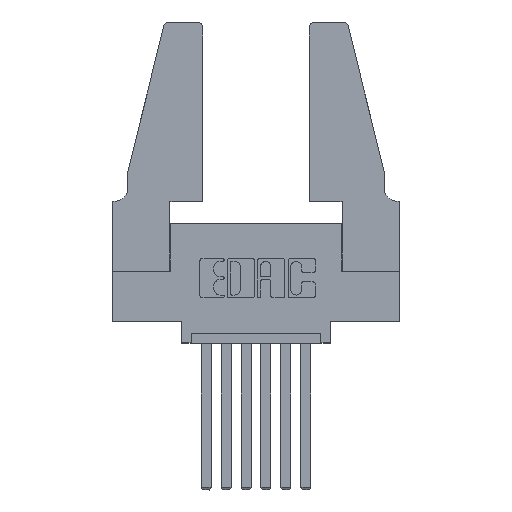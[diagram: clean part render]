
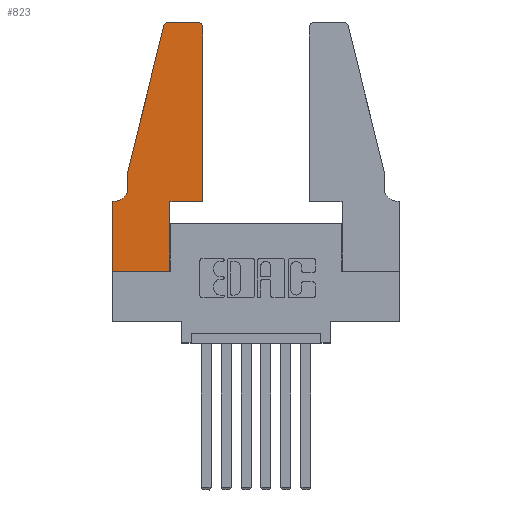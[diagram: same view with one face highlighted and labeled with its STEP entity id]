
A CAD part, top view. The second image highlights one B-rep face of the part: STEP entity #823.
In plain terms, the highlighted planar face has unit normal (0, 0, 1).
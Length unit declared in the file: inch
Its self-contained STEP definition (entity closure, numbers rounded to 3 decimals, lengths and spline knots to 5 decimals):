
#442 = LINE ( 'NONE', #8422, #3242 ) ;
#522 = EDGE_CURVE ( 'NONE', #2364, #3418, #5829, .T. ) ;
#600 = PLANE ( 'NONE',  #9543 ) ;
#605 = EDGE_CURVE ( 'NONE', #1184, #9651, #3217, .T. ) ;
#698 = CARTESIAN_POINT ( 'NONE',  ( 0.4505, 0.35, 0.37 ) ) ;
#705 = DIRECTION ( 'NONE',  ( 1., 0., 0. ) ) ;
#805 = ORIENTED_EDGE ( 'NONE', *, *, #5614, .T. ) ;
#823 = ADVANCED_FACE ( 'NONE', ( #4710 ), #600, .T. ) ;
#920 = CARTESIAN_POINT ( 'NONE',  ( 0.0055, 0.42, 0.37 ) ) ;
#1025 = DIRECTION ( 'NONE',  ( 0., 0., 1. ) ) ;
#1041 = VECTOR ( 'NONE', #3894, 39.37008 ) ;
#1184 = VERTEX_POINT ( 'NONE', #3946 ) ;
#1202 = ORIENTED_EDGE ( 'NONE', *, *, #522, .T. ) ;
#1236 = EDGE_LOOP ( 'NONE', ( #1202, #2286, #8239, #10506, #7059, #2358, #10195, #8709, #805, #8279, #3231, #5158 ) ) ;
#1479 = LINE ( 'NONE', #3176, #9645 ) ;
#1609 = DIRECTION ( 'NONE',  ( -0.239, -0.971, 0. ) ) ;
#1748 = AXIS2_PLACEMENT_3D ( 'NONE', #2645, #4432, #5366 ) ;
#1759 = CARTESIAN_POINT ( 'NONE',  ( 0.0755, 0.5, 0.37 ) ) ;
#1857 = VERTEX_POINT ( 'NONE', #6319 ) ;
#2286 = ORIENTED_EDGE ( 'NONE', *, *, #5593, .T. ) ;
#2358 = ORIENTED_EDGE ( 'NONE', *, *, #8262, .T. ) ;
#2364 = VERTEX_POINT ( 'NONE', #5955 ) ;
#2372 = DIRECTION ( 'NONE',  ( 0., 0., 1. ) ) ;
#2502 = LINE ( 'NONE', #9892, #9300 ) ;
#2555 = CARTESIAN_POINT ( 'NONE',  ( 0.2865, 0., 0.37 ) ) ;
#2618 = CARTESIAN_POINT ( 'NONE',  ( 0.0055, 0.35, 0.37 ) ) ;
#2628 = LINE ( 'NONE', #5241, #9415 ) ;
#2645 = CARTESIAN_POINT ( 'NONE',  ( 0.4205, 1.22, 0.37 ) ) ;
#2779 = VECTOR ( 'NONE', #4278, 39.37008 ) ;
#2802 = CARTESIAN_POINT ( 'NONE',  ( 0.4505, 0.35, 0.37 ) ) ;
#2878 = EDGE_CURVE ( 'NONE', #7506, #5912, #8418, .T. ) ;
#2885 = CARTESIAN_POINT ( 'NONE',  ( 0.284, 1.25, 0.37 ) ) ;
#2950 = EDGE_CURVE ( 'NONE', #1857, #10022, #6340, .T. ) ;
#3176 = CARTESIAN_POINT ( 'NONE',  ( 0., 0., 0.37 ) ) ;
#3217 = LINE ( 'NONE', #698, #2779 ) ;
#3231 = ORIENTED_EDGE ( 'NONE', *, *, #3280, .T. ) ;
#3242 = VECTOR ( 'NONE', #6685, 39.37008 ) ;
#3280 = EDGE_CURVE ( 'NONE', #9651, #7322, #8269, .T. ) ;
#3418 = VERTEX_POINT ( 'NONE', #2885 ) ;
#3425 = CIRCLE ( 'NONE', #10325, 0.03 ) ;
#3571 = VECTOR ( 'NONE', #8111, 39.37008 ) ;
#3894 = DIRECTION ( 'NONE',  ( 0., 1., 0. ) ) ;
#3896 = CARTESIAN_POINT ( 'NONE',  ( 0.4505, 0.35, 0.37 ) ) ;
#3946 = CARTESIAN_POINT ( 'NONE',  ( 0.2865, 0.35, 0.37 ) ) ;
#3966 = DIRECTION ( 'NONE',  ( 1., 0., 0. ) ) ;
#4278 = DIRECTION ( 'NONE',  ( 1., 0., 0. ) ) ;
#4323 = CARTESIAN_POINT ( 'NONE',  ( 0.4505, 1.22, 0.37 ) ) ;
#4432 = DIRECTION ( 'NONE',  ( 0., 0., 1. ) ) ;
#4511 = CARTESIAN_POINT ( 'NONE',  ( 0., 0.35, 0.37 ) ) ;
#4710 = FACE_OUTER_BOUND ( 'NONE', #1236, .T. ) ;
#4759 = VERTEX_POINT ( 'NONE', #4511 ) ;
#5003 = EDGE_CURVE ( 'NONE', #5912, #1857, #442, .T. ) ;
#5158 = ORIENTED_EDGE ( 'NONE', *, *, #9045, .T. ) ;
#5241 = CARTESIAN_POINT ( 'NONE',  ( 0., 0., 0.37 ) ) ;
#5366 = DIRECTION ( 'NONE',  ( 1., 0., 0. ) ) ;
#5539 = VECTOR ( 'NONE', #6517, 39.37008 ) ;
#5593 = EDGE_CURVE ( 'NONE', #3418, #7506, #3425, .T. ) ;
#5614 = EDGE_CURVE ( 'NONE', #10525, #1184, #9784, .T. ) ;
#5745 = CARTESIAN_POINT ( 'NONE',  ( 0.2865, 0.35, 0.37 ) ) ;
#5829 = LINE ( 'NONE', #8240, #5539 ) ;
#5912 = VERTEX_POINT ( 'NONE', #7587 ) ;
#5955 = CARTESIAN_POINT ( 'NONE',  ( 0.4205, 1.25, 0.37 ) ) ;
#6010 = EDGE_CURVE ( 'NONE', #4759, #7731, #1479, .T. ) ;
#6212 = DIRECTION ( 'NONE',  ( -1., 0., 0. ) ) ;
#6319 = CARTESIAN_POINT ( 'NONE',  ( 0.0755, 0.42, 0.37 ) ) ;
#6340 = CIRCLE ( 'NONE', #10141, 0.07 ) ;
#6517 = DIRECTION ( 'NONE',  ( -1., 0., 0. ) ) ;
#6685 = DIRECTION ( 'NONE',  ( 0., -1., 0. ) ) ;
#7049 = CARTESIAN_POINT ( 'NONE',  ( 0., 0., 0.37 ) ) ;
#7059 = ORIENTED_EDGE ( 'NONE', *, *, #2950, .T. ) ;
#7322 = VERTEX_POINT ( 'NONE', #4323 ) ;
#7506 = VERTEX_POINT ( 'NONE', #11003 ) ;
#7587 = CARTESIAN_POINT ( 'NONE',  ( 0.0755, 0.5, 0.37 ) ) ;
#7640 = CIRCLE ( 'NONE', #1748, 0.03 ) ;
#7731 = VERTEX_POINT ( 'NONE', #7049 ) ;
#8111 = DIRECTION ( 'NONE',  ( 0., 1., 0. ) ) ;
#8239 = ORIENTED_EDGE ( 'NONE', *, *, #2878, .T. ) ;
#8240 = CARTESIAN_POINT ( 'NONE',  ( 0.2605, 1.25, 0.37 ) ) ;
#8262 = EDGE_CURVE ( 'NONE', #10022, #4759, #2502, .T. ) ;
#8269 = LINE ( 'NONE', #2802, #3571 ) ;
#8279 = ORIENTED_EDGE ( 'NONE', *, *, #605, .T. ) ;
#8418 = LINE ( 'NONE', #1759, #9513 ) ;
#8422 = CARTESIAN_POINT ( 'NONE',  ( 0.0755, 0.5, 0.37 ) ) ;
#8546 = CARTESIAN_POINT ( 'NONE',  ( 0., 0.35, 0.37 ) ) ;
#8692 = DIRECTION ( 'NONE',  ( 1., 0., 0. ) ) ;
#8709 = ORIENTED_EDGE ( 'NONE', *, *, #10501, .T. ) ;
#9045 = EDGE_CURVE ( 'NONE', #7322, #2364, #7640, .T. ) ;
#9300 = VECTOR ( 'NONE', #10759, 39.37008 ) ;
#9415 = VECTOR ( 'NONE', #705, 39.37008 ) ;
#9513 = VECTOR ( 'NONE', #1609, 39.37008 ) ;
#9543 = AXIS2_PLACEMENT_3D ( 'NONE', #8546, #2372, #8692 ) ;
#9645 = VECTOR ( 'NONE', #10238, 39.37008 ) ;
#9651 = VERTEX_POINT ( 'NONE', #3896 ) ;
#9784 = LINE ( 'NONE', #5745, #1041 ) ;
#9892 = CARTESIAN_POINT ( 'NONE',  ( 0.0755, 0.35, 0.37 ) ) ;
#10022 = VERTEX_POINT ( 'NONE', #2618 ) ;
#10141 = AXIS2_PLACEMENT_3D ( 'NONE', #920, #11470, #6212 ) ;
#10195 = ORIENTED_EDGE ( 'NONE', *, *, #6010, .T. ) ;
#10238 = DIRECTION ( 'NONE',  ( 0., -1., 0. ) ) ;
#10325 = AXIS2_PLACEMENT_3D ( 'NONE', #10731, #1025, #3966 ) ;
#10501 = EDGE_CURVE ( 'NONE', #7731, #10525, #2628, .T. ) ;
#10506 = ORIENTED_EDGE ( 'NONE', *, *, #5003, .T. ) ;
#10525 = VERTEX_POINT ( 'NONE', #2555 ) ;
#10731 = CARTESIAN_POINT ( 'NONE',  ( 0.284, 1.22, 0.37 ) ) ;
#10759 = DIRECTION ( 'NONE',  ( -1., 0., 0. ) ) ;
#11003 = CARTESIAN_POINT ( 'NONE',  ( 0.25487, 1.22718, 0.37 ) ) ;
#11470 = DIRECTION ( 'NONE',  ( 0., 0., -1. ) ) ;
